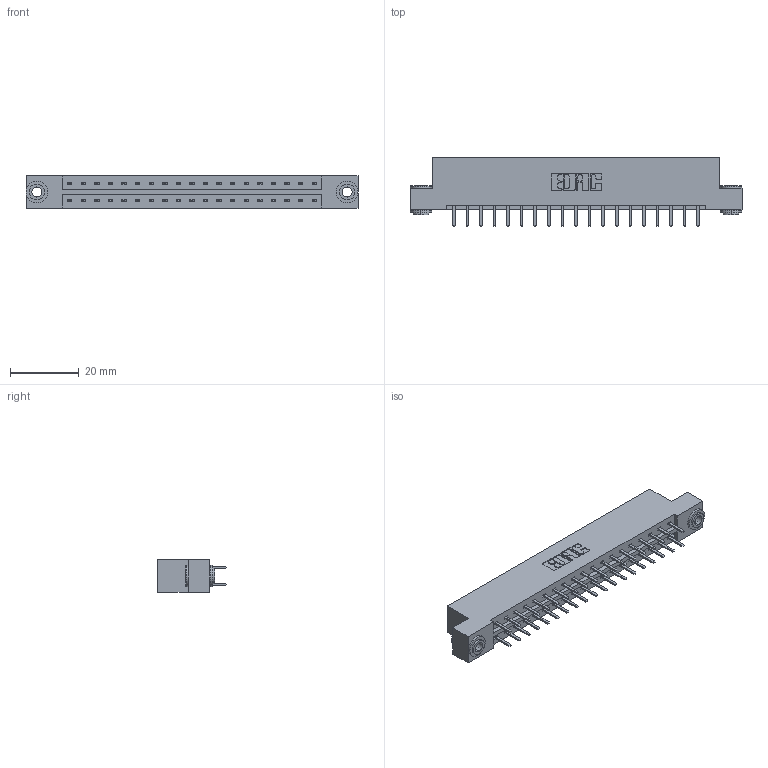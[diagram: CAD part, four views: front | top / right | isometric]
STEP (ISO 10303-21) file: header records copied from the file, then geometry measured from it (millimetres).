
FILE_DESCRIPTION (( 'STEP AP203' ), '1' );
FILE_NAME ('333-038-520-203.STEP', '2018-08-03T03:24:58', ( '' ), ( '' ), 'SwSTEP 2.0', 'SolidWorks 2016', '' );
FILE_SCHEMA (( 'CONFIG_CONTROL_DESIGN' ));
Length unit declared in the file: inch
Products named in the file (4): 333 Part_Flush - .156 Dia - TH; 345-292-001_345-293-120; 345-250-002_345-250-002-102; 333-038-520-203
Assembly tree (41 placements, depth 2):
  333-038-520-203
    333 Part_Flush - .156 Dia - TH
    345-292-001_345-293-120  x38
    345-250-002_345-250-002-102  x2
Bounding box: 96.82 x 20.02 x 9.4 mm (x, y, z)
Volume: 9672.9 mm3; surface area: 11365.2 mm2
Topology: 41 solids, 41 shells, 2280 faces, 6581 edges, 4282 vertices
Faces by surface type: plane 1524, cylinder 748, cone 8
Entity records: 15962 total; most frequent: CARTESIAN_POINT 2661, ORIENTED_EDGE 2578, DIRECTION 2335, EDGE_CURVE 1289, VECTOR 1133, LINE 1133, VERTEX_POINT 854, AXIS2_PLACEMENT_3D 601
